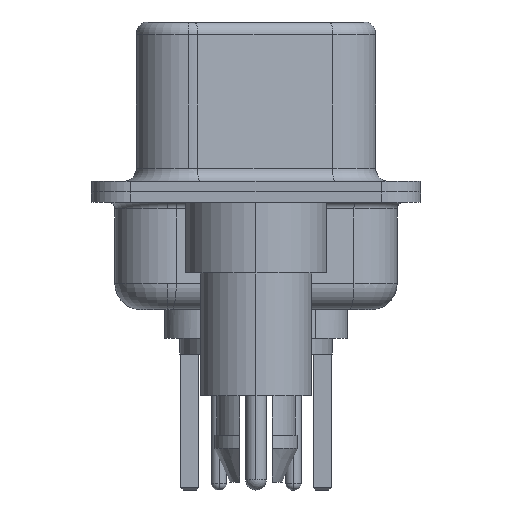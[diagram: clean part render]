
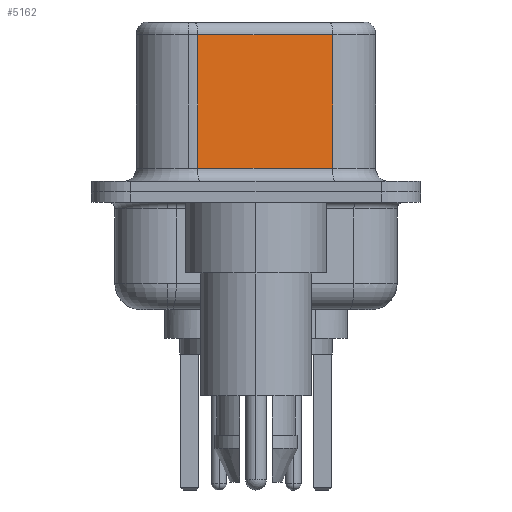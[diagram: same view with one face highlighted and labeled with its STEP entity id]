
A CAD part, left-side view. The second image highlights one B-rep face of the part: STEP entity #5162.
In plain terms, the highlighted planar face has unit normal (-0.985, -0.174, 0).
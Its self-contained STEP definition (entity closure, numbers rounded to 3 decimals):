
#334 = EDGE_CURVE ( 'NONE', #21399, #12668, #1242, .T. ) ;
#856 = AXIS2_PLACEMENT_3D ( 'NONE', #13852, #12220, #1190 ) ;
#1190 = DIRECTION ( 'NONE',  ( -0.174, 0.985, 0. ) ) ;
#1242 = LINE ( 'NONE', #1757, #13566 ) ;
#1757 = CARTESIAN_POINT ( 'NONE',  ( 4.585, -2.927, 6.52 ) ) ;
#1928 = CARTESIAN_POINT ( 'NONE',  ( 3.675, 2.233, 6.02 ) ) ;
#3146 = PLANE ( 'NONE',  #856 ) ;
#3602 = ORIENTED_EDGE ( 'NONE', *, *, #5592, .T. ) ;
#4475 = CARTESIAN_POINT ( 'NONE',  ( 4.585, -2.927, 6.02 ) ) ;
#5050 = CARTESIAN_POINT ( 'NONE',  ( 4.585, -2.927, 6.02 ) ) ;
#5162 = ADVANCED_FACE ( 'NONE', ( #17744 ), #3146, .F. ) ;
#5592 = EDGE_CURVE ( 'NONE', #6509, #12668, #6451, .T. ) ;
#5599 = VECTOR ( 'NONE', #11021, 1000. ) ;
#5929 = VECTOR ( 'NONE', #11429, 1000. ) ;
#6451 = LINE ( 'NONE', #10450, #5929 ) ;
#6509 = VERTEX_POINT ( 'NONE', #9501 ) ;
#8254 = CARTESIAN_POINT ( 'NONE',  ( 4.585, -2.927, 0.9 ) ) ;
#8483 = VECTOR ( 'NONE', #14523, 1000. ) ;
#9501 = CARTESIAN_POINT ( 'NONE',  ( 3.675, 2.233, 0.9 ) ) ;
#9786 = VERTEX_POINT ( 'NONE', #1928 ) ;
#9881 = EDGE_LOOP ( 'NONE', ( #12200, #14204, #18103, #3602 ) ) ;
#10450 = CARTESIAN_POINT ( 'NONE',  ( 4.585, -2.927, 0.9 ) ) ;
#11021 = DIRECTION ( 'NONE',  ( 0., 0., -1. ) ) ;
#11429 = DIRECTION ( 'NONE',  ( 0.174, -0.985, 0. ) ) ;
#12200 = ORIENTED_EDGE ( 'NONE', *, *, #334, .F. ) ;
#12220 = DIRECTION ( 'NONE',  ( 0.985, 0.174, 0. ) ) ;
#12668 = VERTEX_POINT ( 'NONE', #8254 ) ;
#13428 = LINE ( 'NONE', #4475, #8483 ) ;
#13566 = VECTOR ( 'NONE', #15017, 1000. ) ;
#13852 = CARTESIAN_POINT ( 'NONE',  ( 4.585, -2.927, 6.52 ) ) ;
#13954 = EDGE_CURVE ( 'NONE', #9786, #6509, #18481, .T. ) ;
#14011 = EDGE_CURVE ( 'NONE', #21399, #9786, #13428, .T. ) ;
#14204 = ORIENTED_EDGE ( 'NONE', *, *, #14011, .T. ) ;
#14523 = DIRECTION ( 'NONE',  ( -0.174, 0.985, 0. ) ) ;
#15017 = DIRECTION ( 'NONE',  ( 0., 0., -1. ) ) ;
#17744 = FACE_OUTER_BOUND ( 'NONE', #9881, .T. ) ;
#17776 = CARTESIAN_POINT ( 'NONE',  ( 3.675, 2.233, 6.52 ) ) ;
#18103 = ORIENTED_EDGE ( 'NONE', *, *, #13954, .T. ) ;
#18481 = LINE ( 'NONE', #17776, #5599 ) ;
#21399 = VERTEX_POINT ( 'NONE', #5050 ) ;
